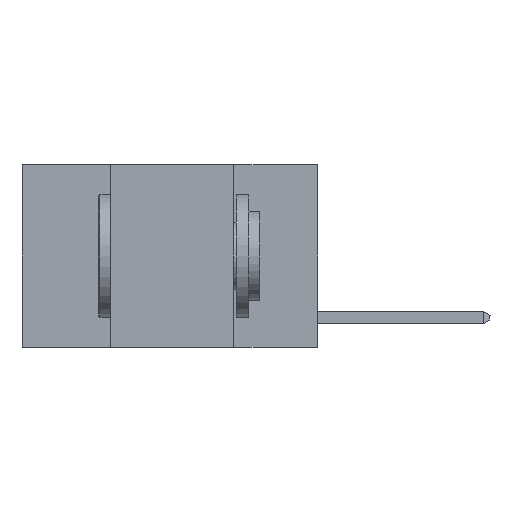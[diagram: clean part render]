
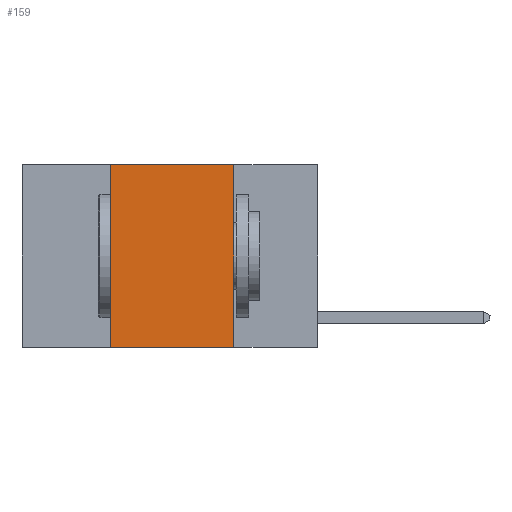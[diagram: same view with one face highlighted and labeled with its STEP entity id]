
A CAD part, left-side view. The second image highlights one B-rep face of the part: STEP entity #159.
In plain terms, the highlighted planar face has unit normal (-1, 0, 0).
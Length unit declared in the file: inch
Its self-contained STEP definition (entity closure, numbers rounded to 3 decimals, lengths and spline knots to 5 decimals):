
#159 = ADVANCED_FACE ( 'NONE', ( #10180 ), #8039, .F. ) ;
#920 = CARTESIAN_POINT ( 'NONE',  ( 0., 0.17, 0. ) ) ;
#1084 = CARTESIAN_POINT ( 'NONE',  ( 0., 0.42, 0. ) ) ;
#1603 = DIRECTION ( 'NONE',  ( 0., -1., 0. ) ) ;
#1694 = DIRECTION ( 'NONE',  ( 0., 0., -1. ) ) ;
#1803 = VECTOR ( 'NONE', #1603, 39.37008 ) ;
#2631 = ORIENTED_EDGE ( 'NONE', *, *, #12102, .T. ) ;
#2646 = VECTOR ( 'NONE', #1694, 39.37008 ) ;
#2983 = LINE ( 'NONE', #6686, #13404 ) ;
#3025 = EDGE_CURVE ( 'NONE', #8539, #7514, #10763, .T. ) ;
#3086 = CARTESIAN_POINT ( 'NONE',  ( 0., 0.42, -0.37 ) ) ;
#3088 = CARTESIAN_POINT ( 'NONE',  ( 0., 0.17, -0.37 ) ) ;
#3341 = EDGE_CURVE ( 'NONE', #7514, #11412, #4660, .T. ) ;
#3485 = ORIENTED_EDGE ( 'NONE', *, *, #3341, .F. ) ;
#4386 = VERTEX_POINT ( 'NONE', #3086 ) ;
#4660 = LINE ( 'NONE', #8983, #2646 ) ;
#4714 = DIRECTION ( 'NONE',  ( 0., 0., -1. ) ) ;
#4761 = LINE ( 'NONE', #1084, #13526 ) ;
#5293 = EDGE_LOOP ( 'NONE', ( #3485, #13133, #12167, #2631 ) ) ;
#5648 = DIRECTION ( 'NONE',  ( 0., -1., 0. ) ) ;
#6406 = AXIS2_PLACEMENT_3D ( 'NONE', #12056, #9842, #4714 ) ;
#6686 = CARTESIAN_POINT ( 'NONE',  ( 0., 0.6, -0.37 ) ) ;
#7514 = VERTEX_POINT ( 'NONE', #920 ) ;
#8039 = PLANE ( 'NONE',  #6406 ) ;
#8539 = VERTEX_POINT ( 'NONE', #12219 ) ;
#8983 = CARTESIAN_POINT ( 'NONE',  ( 0., 0.17, 0. ) ) ;
#9186 = EDGE_CURVE ( 'NONE', #4386, #8539, #4761, .T. ) ;
#9618 = DIRECTION ( 'NONE',  ( 0., 0., 1. ) ) ;
#9842 = DIRECTION ( 'NONE',  ( 1., 0., 0. ) ) ;
#10180 = FACE_OUTER_BOUND ( 'NONE', #5293, .T. ) ;
#10763 = LINE ( 'NONE', #11339, #1803 ) ;
#11339 = CARTESIAN_POINT ( 'NONE',  ( 0., 0.6, 0. ) ) ;
#11412 = VERTEX_POINT ( 'NONE', #3088 ) ;
#12056 = CARTESIAN_POINT ( 'NONE',  ( 0., 0.6, 0. ) ) ;
#12102 = EDGE_CURVE ( 'NONE', #4386, #11412, #2983, .T. ) ;
#12167 = ORIENTED_EDGE ( 'NONE', *, *, #9186, .F. ) ;
#12219 = CARTESIAN_POINT ( 'NONE',  ( 0., 0.42, 0. ) ) ;
#13133 = ORIENTED_EDGE ( 'NONE', *, *, #3025, .F. ) ;
#13404 = VECTOR ( 'NONE', #5648, 39.37008 ) ;
#13526 = VECTOR ( 'NONE', #9618, 39.37008 ) ;
